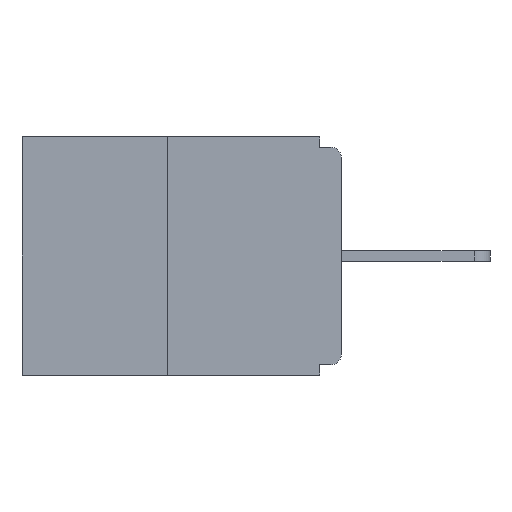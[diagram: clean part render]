
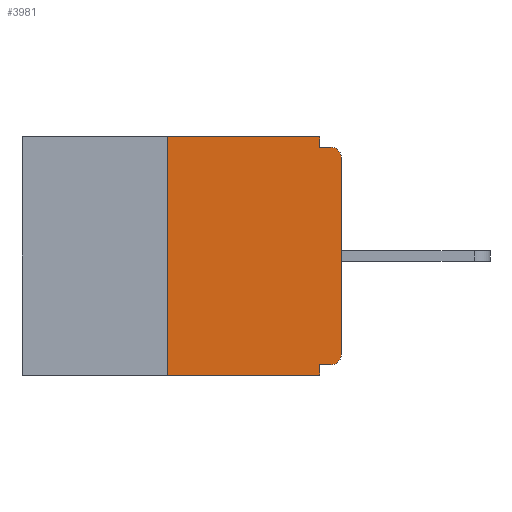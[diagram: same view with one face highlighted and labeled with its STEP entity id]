
A CAD part, left-side view. The second image highlights one B-rep face of the part: STEP entity #3981.
In plain terms, the highlighted planar face has unit normal (-1, 0, 0).
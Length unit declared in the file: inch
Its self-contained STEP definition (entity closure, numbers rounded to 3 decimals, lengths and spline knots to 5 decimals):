
#619 = VECTOR ( 'NONE', #4825, 39.37008 ) ;
#807 = CARTESIAN_POINT ( 'NONE',  ( 0., 0., -0.313 ) ) ;
#990 = LINE ( 'NONE', #2188, #619 ) ;
#1133 = VERTEX_POINT ( 'NONE', #10161 ) ;
#1288 = DIRECTION ( 'NONE',  ( 0., 0., -1. ) ) ;
#1289 = EDGE_LOOP ( 'NONE', ( #4565, #3231, #6677, #2850, #2063, #7246, #2076, #7129, #7328, #2737 ) ) ;
#1406 = DIRECTION ( 'NONE',  ( 0., 0., -1. ) ) ;
#1442 = FACE_OUTER_BOUND ( 'NONE', #1289, .T. ) ;
#1787 = CARTESIAN_POINT ( 'NONE',  ( 0., 0.031, 0. ) ) ;
#1812 = DIRECTION ( 'NONE',  ( 1., 0., 0. ) ) ;
#1995 = VERTEX_POINT ( 'NONE', #807 ) ;
#2063 = ORIENTED_EDGE ( 'NONE', *, *, #3494, .F. ) ;
#2076 = ORIENTED_EDGE ( 'NONE', *, *, #3436, .T. ) ;
#2099 = CARTESIAN_POINT ( 'NONE',  ( 0., 0.031, -0.343 ) ) ;
#2188 = CARTESIAN_POINT ( 'NONE',  ( 0., 0.25, 0. ) ) ;
#2603 = VERTEX_POINT ( 'NONE', #2628 ) ;
#2628 = CARTESIAN_POINT ( 'NONE',  ( 0., 0.25, 0. ) ) ;
#2705 = AXIS2_PLACEMENT_3D ( 'NONE', #10465, #1812, #1406 ) ;
#2737 = ORIENTED_EDGE ( 'NONE', *, *, #4292, .F. ) ;
#2780 = CARTESIAN_POINT ( 'NONE',  ( 0., 0., -0.03 ) ) ;
#2850 = ORIENTED_EDGE ( 'NONE', *, *, #4275, .F. ) ;
#3173 = CARTESIAN_POINT ( 'NONE',  ( 0., 0.46, -0.343 ) ) ;
#3231 = ORIENTED_EDGE ( 'NONE', *, *, #4221, .F. ) ;
#3436 = EDGE_CURVE ( 'NONE', #1995, #10325, #5755, .T. ) ;
#3457 = CARTESIAN_POINT ( 'NONE',  ( 0., 0.031, -0.328 ) ) ;
#3494 = EDGE_CURVE ( 'NONE', #7507, #8284, #4809, .T. ) ;
#3589 = EDGE_CURVE ( 'NONE', #9909, #7685, #4008, .T. ) ;
#3609 = EDGE_CURVE ( 'NONE', #7507, #1995, #3955, .T. ) ;
#3633 = EDGE_CURVE ( 'NONE', #10325, #7685, #3704, .T. ) ;
#3704 = CIRCLE ( 'NONE', #5903, 0.015 ) ;
#3955 = CIRCLE ( 'NONE', #10166, 0.015 ) ;
#3976 = VECTOR ( 'NONE', #7327, 39.37008 ) ;
#3981 = ADVANCED_FACE ( 'NONE', ( #1442 ), #10592, .F. ) ;
#4008 = LINE ( 'NONE', #9245, #3976 ) ;
#4062 = DIRECTION ( 'NONE',  ( 0., -1., 0. ) ) ;
#4190 = DIRECTION ( 'NONE',  ( 0., -1., 0. ) ) ;
#4221 = EDGE_CURVE ( 'NONE', #1133, #2603, #990, .T. ) ;
#4238 = EDGE_CURVE ( 'NONE', #1133, #5089, #5715, .T. ) ;
#4275 = EDGE_CURVE ( 'NONE', #8284, #5089, #10284, .T. ) ;
#4292 = EDGE_CURVE ( 'NONE', #8897, #9909, #6509, .T. ) ;
#4421 = EDGE_CURVE ( 'NONE', #2603, #8897, #7851, .T. ) ;
#4565 = ORIENTED_EDGE ( 'NONE', *, *, #4421, .F. ) ;
#4809 = LINE ( 'NONE', #9662, #4887 ) ;
#4825 = DIRECTION ( 'NONE',  ( 0., 0., 1. ) ) ;
#4887 = VECTOR ( 'NONE', #6611, 39.37008 ) ;
#5089 = VERTEX_POINT ( 'NONE', #6882 ) ;
#5537 = VECTOR ( 'NONE', #6690, 39.37008 ) ;
#5613 = CARTESIAN_POINT ( 'NONE',  ( 0., 0.015, -0.015 ) ) ;
#5715 = LINE ( 'NONE', #3173, #10610 ) ;
#5755 = LINE ( 'NONE', #6617, #5537 ) ;
#5903 = AXIS2_PLACEMENT_3D ( 'NONE', #8607, #8618, #8596 ) ;
#6509 = LINE ( 'NONE', #10518, #8406 ) ;
#6611 = DIRECTION ( 'NONE',  ( 0., 1., 0. ) ) ;
#6617 = CARTESIAN_POINT ( 'NONE',  ( 0., 0., 0. ) ) ;
#6637 = CARTESIAN_POINT ( 'NONE',  ( 0., 0.015, -0.328 ) ) ;
#6677 = ORIENTED_EDGE ( 'NONE', *, *, #4238, .T. ) ;
#6690 = DIRECTION ( 'NONE',  ( 0., 0., 1. ) ) ;
#6882 = CARTESIAN_POINT ( 'NONE',  ( 0., 0.031, -0.343 ) ) ;
#6961 = CARTESIAN_POINT ( 'NONE',  ( 0., 0.46, 0. ) ) ;
#6967 = VECTOR ( 'NONE', #1288, 39.37008 ) ;
#7129 = ORIENTED_EDGE ( 'NONE', *, *, #3633, .T. ) ;
#7246 = ORIENTED_EDGE ( 'NONE', *, *, #3609, .T. ) ;
#7327 = DIRECTION ( 'NONE',  ( 0., -1., 0. ) ) ;
#7328 = ORIENTED_EDGE ( 'NONE', *, *, #3589, .F. ) ;
#7507 = VERTEX_POINT ( 'NONE', #6637 ) ;
#7685 = VERTEX_POINT ( 'NONE', #5613 ) ;
#7851 = LINE ( 'NONE', #6961, #9411 ) ;
#8284 = VERTEX_POINT ( 'NONE', #3457 ) ;
#8406 = VECTOR ( 'NONE', #10573, 39.37008 ) ;
#8437 = CARTESIAN_POINT ( 'NONE',  ( 0., 0.031, -0.015 ) ) ;
#8596 = DIRECTION ( 'NONE',  ( 0., 0., -1. ) ) ;
#8607 = CARTESIAN_POINT ( 'NONE',  ( 0., 0.015, -0.03 ) ) ;
#8618 = DIRECTION ( 'NONE',  ( -1., 0., 0. ) ) ;
#8897 = VERTEX_POINT ( 'NONE', #1787 ) ;
#9245 = CARTESIAN_POINT ( 'NONE',  ( 0., 0., -0.015 ) ) ;
#9411 = VECTOR ( 'NONE', #4190, 39.37008 ) ;
#9662 = CARTESIAN_POINT ( 'NONE',  ( 0., 0., -0.328 ) ) ;
#9819 = DIRECTION ( 'NONE',  ( 0., 0., -1. ) ) ;
#9827 = DIRECTION ( 'NONE',  ( -1., 0., 0. ) ) ;
#9831 = CARTESIAN_POINT ( 'NONE',  ( 0., 0.015, -0.313 ) ) ;
#9909 = VERTEX_POINT ( 'NONE', #8437 ) ;
#10161 = CARTESIAN_POINT ( 'NONE',  ( 0., 0.25, -0.343 ) ) ;
#10166 = AXIS2_PLACEMENT_3D ( 'NONE', #9831, #9827, #9819 ) ;
#10284 = LINE ( 'NONE', #2099, #6967 ) ;
#10325 = VERTEX_POINT ( 'NONE', #2780 ) ;
#10465 = CARTESIAN_POINT ( 'NONE',  ( 0., 0.46, 0. ) ) ;
#10518 = CARTESIAN_POINT ( 'NONE',  ( 0., 0.031, 0. ) ) ;
#10573 = DIRECTION ( 'NONE',  ( 0., 0., -1. ) ) ;
#10592 = PLANE ( 'NONE',  #2705 ) ;
#10610 = VECTOR ( 'NONE', #4062, 39.37008 ) ;
